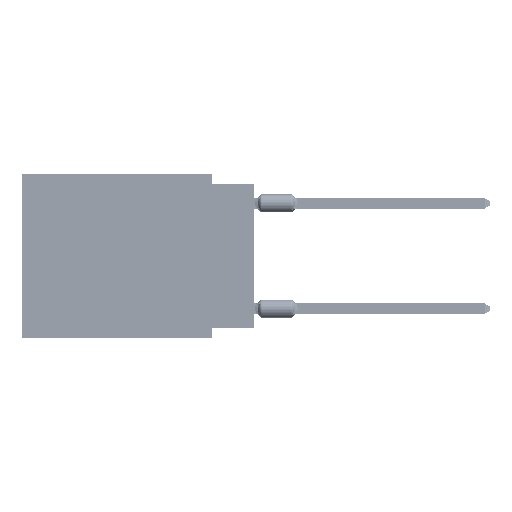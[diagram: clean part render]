
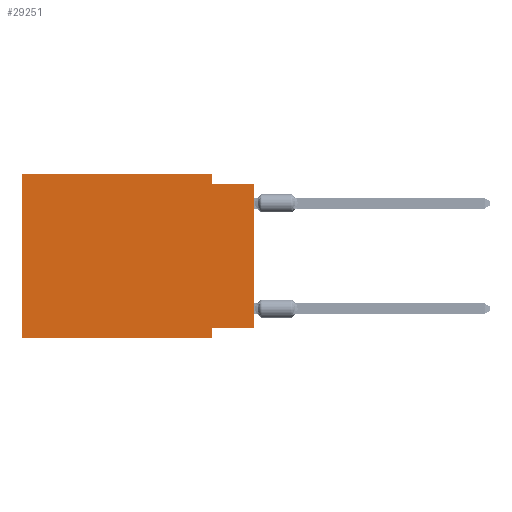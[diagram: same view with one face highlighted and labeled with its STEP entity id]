
A CAD part, left-side view. The second image highlights one B-rep face of the part: STEP entity #29251.
In plain terms, the highlighted planar face has unit normal (-1, 0, 0).
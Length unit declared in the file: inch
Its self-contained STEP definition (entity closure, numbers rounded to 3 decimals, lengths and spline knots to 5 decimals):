
#185 = CARTESIAN_POINT ( 'NONE',  ( 0., 0.55, -0.39 ) ) ;
#1093 = LINE ( 'NONE', #20661, #74311 ) ;
#2670 = ORIENTED_EDGE ( 'NONE', *, *, #70447, .F. ) ;
#5061 = VERTEX_POINT ( 'NONE', #70441 ) ;
#6489 = CARTESIAN_POINT ( 'NONE',  ( 0., 0.1, -0.365 ) ) ;
#7149 = VECTOR ( 'NONE', #84883, 39.37008 ) ;
#7482 = LINE ( 'NONE', #34406, #24387 ) ;
#7659 = EDGE_CURVE ( 'NONE', #30827, #22873, #45357, .T. ) ;
#10121 = ORIENTED_EDGE ( 'NONE', *, *, #7659, .T. ) ;
#12934 = FACE_OUTER_BOUND ( 'NONE', #29272, .T. ) ;
#15246 = VECTOR ( 'NONE', #19682, 39.37008 ) ;
#15930 = DIRECTION ( 'NONE',  ( 0., 0., -1. ) ) ;
#16776 = ORIENTED_EDGE ( 'NONE', *, *, #70761, .F. ) ;
#17159 = CARTESIAN_POINT ( 'NONE',  ( 0., 0.1, -0.39 ) ) ;
#19021 = CARTESIAN_POINT ( 'NONE',  ( 0., 0.55, 0. ) ) ;
#19057 = EDGE_CURVE ( 'NONE', #48854, #57174, #7482, .T. ) ;
#19682 = DIRECTION ( 'NONE',  ( 0., -1., 0. ) ) ;
#20661 = CARTESIAN_POINT ( 'NONE',  ( 0., 0., -0.365 ) ) ;
#21090 = DIRECTION ( 'NONE',  ( 0., 1., 0. ) ) ;
#22873 = VERTEX_POINT ( 'NONE', #56904 ) ;
#23869 = VECTOR ( 'NONE', #84134, 39.37008 ) ;
#24096 = DIRECTION ( 'NONE',  ( 0., 0., -1. ) ) ;
#24252 = AXIS2_PLACEMENT_3D ( 'NONE', #19021, #52005, #37698 ) ;
#24387 = VECTOR ( 'NONE', #29178, 39.37008 ) ;
#26207 = LINE ( 'NONE', #79173, #15246 ) ;
#27223 = EDGE_CURVE ( 'NONE', #5061, #22873, #26207, .T. ) ;
#29178 = DIRECTION ( 'NONE',  ( 0., -1., 0. ) ) ;
#29251 = ADVANCED_FACE ( 'NONE', ( #12934 ), #78078, .F. ) ;
#29272 = EDGE_LOOP ( 'NONE', ( #10121, #39826, #59162, #63367, #40239, #70887, #16776, #2670 ) ) ;
#29981 = VECTOR ( 'NONE', #24096, 39.37008 ) ;
#29990 = CARTESIAN_POINT ( 'NONE',  ( 0., 0.1, 0. ) ) ;
#30827 = VERTEX_POINT ( 'NONE', #36337 ) ;
#33468 = LINE ( 'NONE', #61650, #73690 ) ;
#34406 = CARTESIAN_POINT ( 'NONE',  ( 0., 0.55, 0. ) ) ;
#36337 = CARTESIAN_POINT ( 'NONE',  ( 0., 0., -0.365 ) ) ;
#37698 = DIRECTION ( 'NONE',  ( 0., 0., -1. ) ) ;
#39721 = CARTESIAN_POINT ( 'NONE',  ( 0., 0., 0. ) ) ;
#39826 = ORIENTED_EDGE ( 'NONE', *, *, #27223, .F. ) ;
#40239 = ORIENTED_EDGE ( 'NONE', *, *, #84479, .F. ) ;
#45357 = LINE ( 'NONE', #39721, #7149 ) ;
#45456 = LINE ( 'NONE', #57639, #23869 ) ;
#48854 = VERTEX_POINT ( 'NONE', #54668 ) ;
#52005 = DIRECTION ( 'NONE',  ( 1., 0., 0. ) ) ;
#54570 = EDGE_CURVE ( 'NONE', #58133, #69590, #45456, .T. ) ;
#54668 = CARTESIAN_POINT ( 'NONE',  ( 0., 0.55, 0. ) ) ;
#55422 = LINE ( 'NONE', #75404, #58457 ) ;
#56904 = CARTESIAN_POINT ( 'NONE',  ( 0., 0., -0.025 ) ) ;
#57174 = VERTEX_POINT ( 'NONE', #29990 ) ;
#57308 = VERTEX_POINT ( 'NONE', #6489 ) ;
#57639 = CARTESIAN_POINT ( 'NONE',  ( 0., 0.55, -0.39 ) ) ;
#58133 = VERTEX_POINT ( 'NONE', #185 ) ;
#58457 = VECTOR ( 'NONE', #15930, 39.37008 ) ;
#59162 = ORIENTED_EDGE ( 'NONE', *, *, #79740, .F. ) ;
#61650 = CARTESIAN_POINT ( 'NONE',  ( 0., 0.55, 0. ) ) ;
#63367 = ORIENTED_EDGE ( 'NONE', *, *, #19057, .F. ) ;
#69590 = VERTEX_POINT ( 'NONE', #71717 ) ;
#70441 = CARTESIAN_POINT ( 'NONE',  ( 0., 0.1, -0.025 ) ) ;
#70447 = EDGE_CURVE ( 'NONE', #30827, #57308, #1093, .T. ) ;
#70761 = EDGE_CURVE ( 'NONE', #57308, #69590, #76635, .T. ) ;
#70887 = ORIENTED_EDGE ( 'NONE', *, *, #54570, .T. ) ;
#71717 = CARTESIAN_POINT ( 'NONE',  ( 0., 0.1, -0.39 ) ) ;
#73690 = VECTOR ( 'NONE', #80333, 39.37008 ) ;
#74311 = VECTOR ( 'NONE', #21090, 39.37008 ) ;
#75404 = CARTESIAN_POINT ( 'NONE',  ( 0., 0.1, 0. ) ) ;
#76635 = LINE ( 'NONE', #17159, #29981 ) ;
#78078 = PLANE ( 'NONE',  #24252 ) ;
#79173 = CARTESIAN_POINT ( 'NONE',  ( 0., 0., -0.025 ) ) ;
#79740 = EDGE_CURVE ( 'NONE', #57174, #5061, #55422, .T. ) ;
#80333 = DIRECTION ( 'NONE',  ( 0., 0., 1. ) ) ;
#84134 = DIRECTION ( 'NONE',  ( 0., -1., 0. ) ) ;
#84479 = EDGE_CURVE ( 'NONE', #58133, #48854, #33468, .T. ) ;
#84883 = DIRECTION ( 'NONE',  ( 0., 0., 1. ) ) ;
